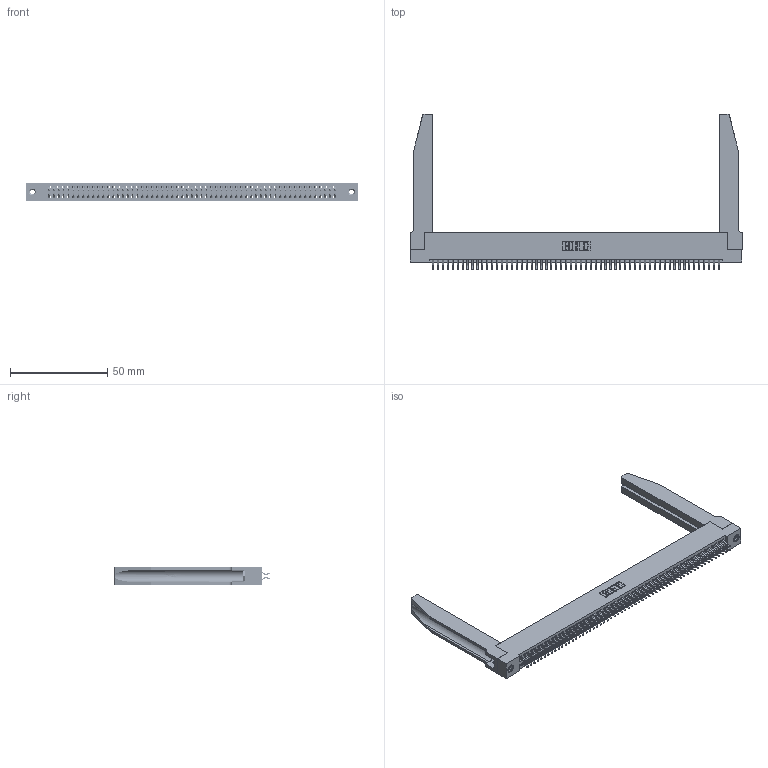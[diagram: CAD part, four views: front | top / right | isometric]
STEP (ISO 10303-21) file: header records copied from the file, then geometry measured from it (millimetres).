
FILE_DESCRIPTION (( 'STEP AP203' ), '1' );
FILE_NAME ('395-118-556-278.STEP', '2019-10-28T01:29:15', ( '' ), ( '' ), 'SwSTEP 2.0', 'SolidWorks 2016', '' );
FILE_SCHEMA (( 'CONFIG_CONTROL_DESIGN' ));
Length unit declared in the file: inch
Products named in the file (5): 395-118-556-278; 345 Part_Flush Mounting Lugs - 0.156 Dia-TH; 345-292-001_556 Tail; 345-250-001_345-250-001-102; 345-220-078_345-220-078
Assembly tree (123 placements, depth 2):
  395-118-556-278
    345 Part_Flush Mounting Lugs - 0.156 Dia-TH
    345-292-001_556 Tail  x118
    345-250-001_345-250-001-102  x2
    345-220-078_345-220-078  x2
Bounding box: 171.09 x 80.2 x 9.4 mm (x, y, z)
Volume: 24543.8 mm3; surface area: 31858.3 mm2
Topology: 123 solids, 123 shells, 6968 faces, 20655 edges, 13602 vertices
Faces by surface type: plane 4588, cylinder 2328, bspline 36, cone 12, torus 4
Entity records: 48964 total; most frequent: CARTESIAN_POINT 9123, ORIENTED_EDGE 7942, DIRECTION 7005, EDGE_CURVE 3971, LINE 3501, VECTOR 3501, VERTEX_POINT 2640, AXIS2_PLACEMENT_3D 1752
